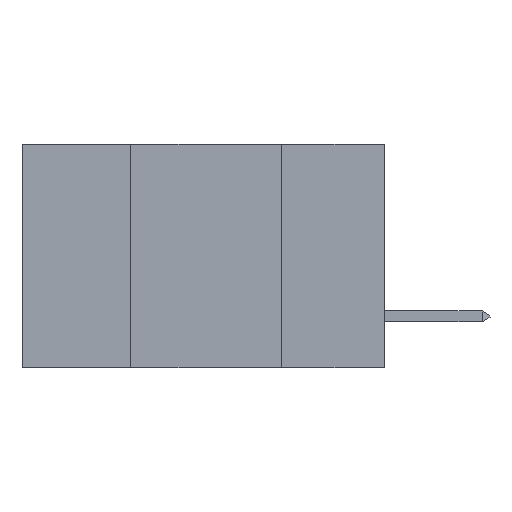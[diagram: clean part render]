
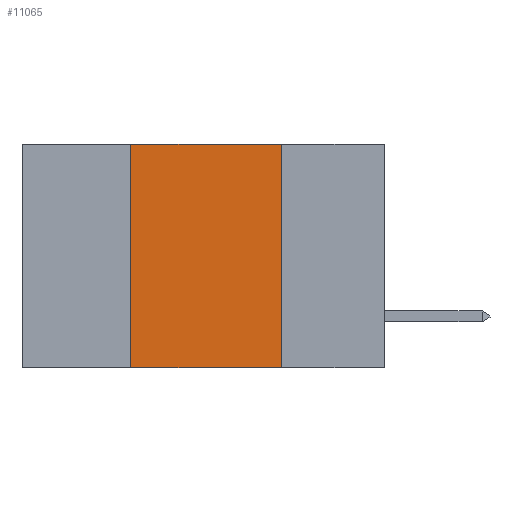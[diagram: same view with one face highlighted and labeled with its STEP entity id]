
A CAD part, left-side view. The second image highlights one B-rep face of the part: STEP entity #11065.
In plain terms, the highlighted planar face has unit normal (-1, 0, 0).
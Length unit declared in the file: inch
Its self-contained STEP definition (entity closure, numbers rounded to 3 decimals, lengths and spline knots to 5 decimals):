
#155 = VERTEX_POINT ( 'NONE', #9058 ) ;
#256 = EDGE_CURVE ( 'NONE', #21270, #10819, #3240, .T. ) ;
#688 = VECTOR ( 'NONE', #23291, 39.37008 ) ;
#738 = CARTESIAN_POINT ( 'NONE',  ( 0., 0.17, -0.37 ) ) ;
#1990 = FACE_OUTER_BOUND ( 'NONE', #23578, .T. ) ;
#3160 = CARTESIAN_POINT ( 'NONE',  ( 0., 0.6, -0.37 ) ) ;
#3240 = LINE ( 'NONE', #14981, #18541 ) ;
#3891 = DIRECTION ( 'NONE',  ( 0., 0., 1. ) ) ;
#4065 = EDGE_CURVE ( 'NONE', #15460, #10819, #5114, .T. ) ;
#4071 = CARTESIAN_POINT ( 'NONE',  ( 0., 0.42, -0.37 ) ) ;
#5114 = LINE ( 'NONE', #3160, #688 ) ;
#5776 = ORIENTED_EDGE ( 'NONE', *, *, #8109, .F. ) ;
#8109 = EDGE_CURVE ( 'NONE', #155, #21270, #14585, .T. ) ;
#8850 = CARTESIAN_POINT ( 'NONE',  ( 0., 0.6, 0. ) ) ;
#9058 = CARTESIAN_POINT ( 'NONE',  ( 0., 0.42, 0. ) ) ;
#10786 = PLANE ( 'NONE',  #19140 ) ;
#10819 = VERTEX_POINT ( 'NONE', #738 ) ;
#11065 = ADVANCED_FACE ( 'NONE', ( #1990 ), #10786, .F. ) ;
#12604 = VECTOR ( 'NONE', #3891, 39.37008 ) ;
#12649 = DIRECTION ( 'NONE',  ( 0., 0., -1. ) ) ;
#13744 = CARTESIAN_POINT ( 'NONE',  ( 0., 0.17, 0. ) ) ;
#14585 = LINE ( 'NONE', #20445, #23543 ) ;
#14981 = CARTESIAN_POINT ( 'NONE',  ( 0., 0.17, 0. ) ) ;
#15164 = DIRECTION ( 'NONE',  ( 0., 0., -1. ) ) ;
#15460 = VERTEX_POINT ( 'NONE', #4071 ) ;
#16186 = ORIENTED_EDGE ( 'NONE', *, *, #21734, .F. ) ;
#16829 = CARTESIAN_POINT ( 'NONE',  ( 0., 0.42, 0. ) ) ;
#18541 = VECTOR ( 'NONE', #15164, 39.37008 ) ;
#19140 = AXIS2_PLACEMENT_3D ( 'NONE', #8850, #23421, #12649 ) ;
#19873 = ORIENTED_EDGE ( 'NONE', *, *, #256, .F. ) ;
#20445 = CARTESIAN_POINT ( 'NONE',  ( 0., 0.6, 0. ) ) ;
#20978 = ORIENTED_EDGE ( 'NONE', *, *, #4065, .T. ) ;
#21270 = VERTEX_POINT ( 'NONE', #13744 ) ;
#21734 = EDGE_CURVE ( 'NONE', #15460, #155, #22731, .T. ) ;
#22225 = DIRECTION ( 'NONE',  ( 0., -1., 0. ) ) ;
#22731 = LINE ( 'NONE', #16829, #12604 ) ;
#23291 = DIRECTION ( 'NONE',  ( 0., -1., 0. ) ) ;
#23421 = DIRECTION ( 'NONE',  ( 1., 0., 0. ) ) ;
#23543 = VECTOR ( 'NONE', #22225, 39.37008 ) ;
#23578 = EDGE_LOOP ( 'NONE', ( #19873, #5776, #16186, #20978 ) ) ;
